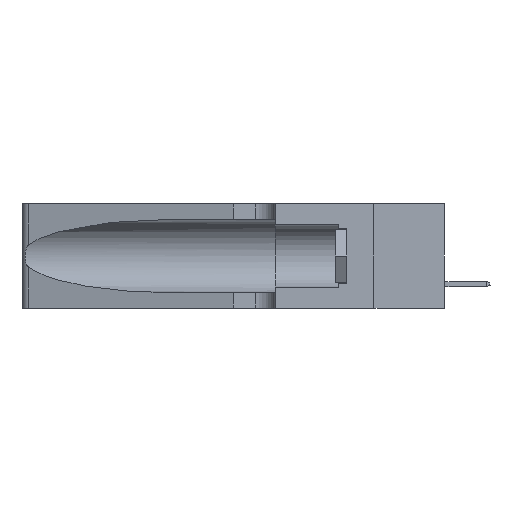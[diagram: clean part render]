
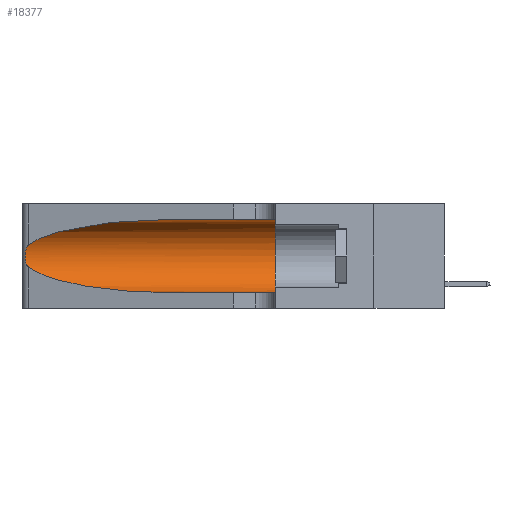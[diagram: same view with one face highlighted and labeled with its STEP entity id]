
A CAD part, left-side view. The second image highlights one B-rep face of the part: STEP entity #18377.
In plain terms, the highlighted cylindrical face has radius 3.308 mm (diameter 6.617 mm), a partial arc.
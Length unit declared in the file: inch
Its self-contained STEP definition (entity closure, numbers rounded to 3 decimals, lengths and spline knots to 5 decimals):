
#311 = EDGE_CURVE ( 'NONE', #24616, #17453, #23996, .T. ) ;
#1564 = VERTEX_POINT ( 'NONE', #5499 ) ;
#2900 = CARTESIAN_POINT ( 'NONE',  ( 0.25639, 1.23184, 0.21858 ) ) ;
#3012 = CARTESIAN_POINT ( 'NONE',  ( 0.25555, 1.22993, 0.14849 ) ) ;
#3129 = CARTESIAN_POINT ( 'NONE',  ( 0.25487, 1.22718, 0.14631 ) ) ;
#4040 = LINE ( 'NONE', #16801, #29460 ) ;
#4127 = ORIENTED_EDGE ( 'NONE', *, *, #13509, .T. ) ;
#5466 = EDGE_CURVE ( 'NONE', #24616, #24600, #20393, .T. ) ;
#5499 = CARTESIAN_POINT ( 'NONE',  ( 0.1305, 0.35, 0.05475 ) ) ;
#5552 = CARTESIAN_POINT ( 'NONE',  ( 0.1305, 0.72297, 0.31525 ) ) ;
#5616 = CARTESIAN_POINT ( 'NONE',  ( 0.25856, 1.23593, 0.16098 ) ) ;
#6139 = DIRECTION ( 'NONE',  ( 0., 0., 1. ) ) ;
#6361 = CARTESIAN_POINT ( 'NONE',  ( 0.1305, 1.61858, 0.31525 ) ) ;
#6520 = EDGE_CURVE ( 'NONE', #17453, #1564, #12409, .T. ) ;
#6797 = DIRECTION ( 'NONE',  ( 0., -1., 0. ) ) ;
#6828 = CARTESIAN_POINT ( 'NONE',  ( 0.1305, 0.35, 0.185 ) ) ;
#7365 = CARTESIAN_POINT ( 'NONE',  ( 0.18966, 0.96281, 0.05475 ) ) ;
#7652 = B_SPLINE_CURVE_WITH_KNOTS ( 'NONE', 3,
 ( #22370, #17842, #2900, #24842, #10282, #15273, #7886, #10485, #22561, #5616, #7701, #15494, #3012, #3129 ),
 .UNSPECIFIED., .F., .F.,
 ( 4, 2, 2, 2, 2, 2, 4 ),
 ( 0., 0.00027, 0.00053, 0.00107, 0.0016, 0.00187, 0.00214 ),
 .UNSPECIFIED. ) ;
#7701 = CARTESIAN_POINT ( 'NONE',  ( 0.25789, 1.23486, 0.15765 ) ) ;
#7864 = DIRECTION ( 'NONE',  ( 0., -1., 0. ) ) ;
#7886 = CARTESIAN_POINT ( 'NONE',  ( 0.26075, 1.23896, 0.19203 ) ) ;
#7921 = CARTESIAN_POINT ( 'NONE',  ( 0.25487, 1.22718, 0.14631 ) ) ;
#8280 = CARTESIAN_POINT ( 'NONE',  ( 0.25487, 1.22718, 0.22369 ) ) ;
#8634 = CARTESIAN_POINT ( 'NONE',  ( 0.18966, 0.96281, 0.31525 ) ) ;
#9624 = CARTESIAN_POINT ( 'NONE',  ( 0.1305, 0.72297, 0.05475 ) ) ;
#10132 = VECTOR ( 'NONE', #16769, 39.37008 ) ;
#10282 = CARTESIAN_POINT ( 'NONE',  ( 0.25854, 1.2359, 0.20912 ) ) ;
#10485 = CARTESIAN_POINT ( 'NONE',  ( 0.26075, 1.23896, 0.178 ) ) ;
#10901 = AXIS2_PLACEMENT_3D ( 'NONE', #6828, #26516, #6139 ) ;
#10991 = EDGE_LOOP ( 'NONE', ( #31230, #20532, #4127, #15241, #28599, #19430 ) ) ;
#12409 = CIRCLE ( 'NONE', #10901, 0.13025 ) ;
#13509 = EDGE_CURVE ( 'NONE', #24731, #27061, #15695, .T. ) ;
#15241 = ORIENTED_EDGE ( 'NONE', *, *, #25109, .T. ) ;
#15273 = CARTESIAN_POINT ( 'NONE',  ( 0.26018, 1.23835, 0.19895 ) ) ;
#15494 = CARTESIAN_POINT ( 'NONE',  ( 0.25639, 1.23186, 0.15144 ) ) ;
#15695 =( BOUNDED_CURVE ( )  B_SPLINE_CURVE ( 3, ( #19366, #29600, #7365, #9624 ),
 .UNSPECIFIED., .F., .T. ) 
 B_SPLINE_CURVE_WITH_KNOTS ( ( 4, 4 ),
 ( 3.44316, 4.71239 ),
 .UNSPECIFIED. ) 
 CURVE ( )  GEOMETRIC_REPRESENTATION_ITEM ( )  RATIONAL_B_SPLINE_CURVE ( ( 1., 0.87, 0.87, 1. ) ) 
 REPRESENTATION_ITEM ( '' )  );
#16017 = CARTESIAN_POINT ( 'NONE',  ( 0.25487, 1.22718, 0.22369 ) ) ;
#16769 = DIRECTION ( 'NONE',  ( 0., -1., 0. ) ) ;
#16801 = CARTESIAN_POINT ( 'NONE',  ( 0.1305, 1.61858, 0.05475 ) ) ;
#16908 = CARTESIAN_POINT ( 'NONE',  ( 0.1305, 0.72297, 0.05475 ) ) ;
#17453 = VERTEX_POINT ( 'NONE', #22587 ) ;
#17692 = DIRECTION ( 'NONE',  ( 0., 0., -1. ) ) ;
#17842 = CARTESIAN_POINT ( 'NONE',  ( 0.25555, 1.22994, 0.2215 ) ) ;
#18256 = CARTESIAN_POINT ( 'NONE',  ( 0.2373, 1.15595, 0.28018 ) ) ;
#18377 = ADVANCED_FACE ( 'NONE', ( #28473 ), #19937, .F. ) ;
#19366 = CARTESIAN_POINT ( 'NONE',  ( 0.25487, 1.22718, 0.14631 ) ) ;
#19430 = ORIENTED_EDGE ( 'NONE', *, *, #311, .F. ) ;
#19937 = CYLINDRICAL_SURFACE ( 'NONE', #26089, 0.13025 ) ;
#20393 =( BOUNDED_CURVE ( )  B_SPLINE_CURVE ( 3, ( #20826, #8634, #18256, #16017 ),
 .UNSPECIFIED., .F., .T. ) 
 B_SPLINE_CURVE_WITH_KNOTS ( ( 4, 4 ),
 ( 1.5708, 2.84003 ),
 .UNSPECIFIED. ) 
 CURVE ( )  GEOMETRIC_REPRESENTATION_ITEM ( )  RATIONAL_B_SPLINE_CURVE ( ( 1., 0.87, 0.87, 1. ) ) 
 REPRESENTATION_ITEM ( '' )  );
#20532 = ORIENTED_EDGE ( 'NONE', *, *, #28401, .T. ) ;
#20826 = CARTESIAN_POINT ( 'NONE',  ( 0.1305, 0.72297, 0.31525 ) ) ;
#22370 = CARTESIAN_POINT ( 'NONE',  ( 0.25487, 1.22718, 0.22369 ) ) ;
#22561 = CARTESIAN_POINT ( 'NONE',  ( 0.26017, 1.23833, 0.17102 ) ) ;
#22587 = CARTESIAN_POINT ( 'NONE',  ( 0.1305, 0.35, 0.31525 ) ) ;
#23996 = LINE ( 'NONE', #6361, #10132 ) ;
#24600 = VERTEX_POINT ( 'NONE', #8280 ) ;
#24616 = VERTEX_POINT ( 'NONE', #5552 ) ;
#24731 = VERTEX_POINT ( 'NONE', #7921 ) ;
#24842 = CARTESIAN_POINT ( 'NONE',  ( 0.25787, 1.23484, 0.2124 ) ) ;
#25109 = EDGE_CURVE ( 'NONE', #27061, #1564, #4040, .T. ) ;
#26089 = AXIS2_PLACEMENT_3D ( 'NONE', #27807, #7864, #17692 ) ;
#26516 = DIRECTION ( 'NONE',  ( 0., 1., 0. ) ) ;
#27061 = VERTEX_POINT ( 'NONE', #16908 ) ;
#27807 = CARTESIAN_POINT ( 'NONE',  ( 0.1305, 1.61858, 0.185 ) ) ;
#28401 = EDGE_CURVE ( 'NONE', #24600, #24731, #7652, .T. ) ;
#28473 = FACE_OUTER_BOUND ( 'NONE', #10991, .T. ) ;
#28599 = ORIENTED_EDGE ( 'NONE', *, *, #6520, .F. ) ;
#29460 = VECTOR ( 'NONE', #6797, 39.37008 ) ;
#29600 = CARTESIAN_POINT ( 'NONE',  ( 0.2373, 1.15595, 0.08982 ) ) ;
#31230 = ORIENTED_EDGE ( 'NONE', *, *, #5466, .T. ) ;
